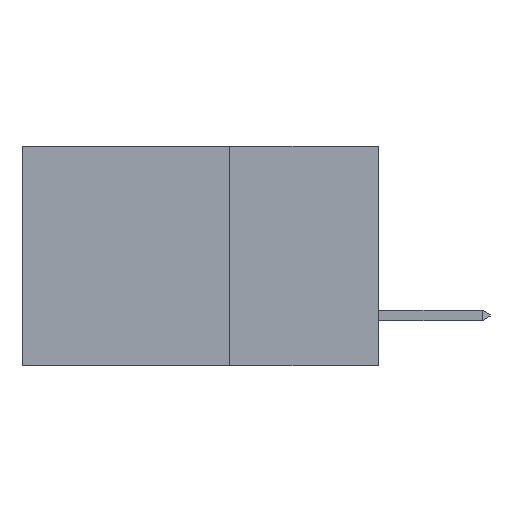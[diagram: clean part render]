
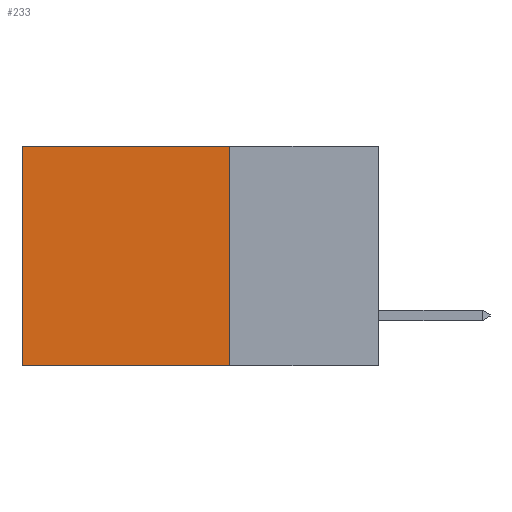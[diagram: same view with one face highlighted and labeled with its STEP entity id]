
A CAD part, left-side view. The second image highlights one B-rep face of the part: STEP entity #233.
In plain terms, the highlighted planar face has unit normal (-1, 0, 0).
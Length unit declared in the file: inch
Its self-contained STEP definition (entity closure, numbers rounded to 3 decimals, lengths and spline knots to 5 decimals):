
#233 = ADVANCED_FACE ( 'NONE', ( #6639 ), #3159, .F. ) ;
#832 = LINE ( 'NONE', #1231, #11042 ) ;
#1231 = CARTESIAN_POINT ( 'NONE',  ( 0.298, 0.25, 0. ) ) ;
#2333 = DIRECTION ( 'NONE',  ( 1., 0., 0. ) ) ;
#2542 = EDGE_LOOP ( 'NONE', ( #14086, #16759, #12512, #13040 ) ) ;
#3117 = LINE ( 'NONE', #8276, #12896 ) ;
#3159 = PLANE ( 'NONE',  #7513 ) ;
#3328 = CARTESIAN_POINT ( 'NONE',  ( 0.298, 0.25, 0. ) ) ;
#3473 = DIRECTION ( 'NONE',  ( 0., 0., -1. ) ) ;
#3909 = LINE ( 'NONE', #15933, #10576 ) ;
#3945 = DIRECTION ( 'NONE',  ( 0., 0., -1. ) ) ;
#4232 = CARTESIAN_POINT ( 'NONE',  ( 0.298, 0.6, 0. ) ) ;
#5231 = EDGE_CURVE ( 'NONE', #8974, #6561, #3909, .T. ) ;
#5378 = VECTOR ( 'NONE', #3473, 39.37008 ) ;
#5754 = EDGE_CURVE ( 'NONE', #14826, #6561, #15957, .T. ) ;
#6089 = CARTESIAN_POINT ( 'NONE',  ( 0.298, 0.25, -0.37 ) ) ;
#6561 = VERTEX_POINT ( 'NONE', #13913 ) ;
#6639 = FACE_OUTER_BOUND ( 'NONE', #2542, .T. ) ;
#7513 = AXIS2_PLACEMENT_3D ( 'NONE', #3328, #2333, #3945 ) ;
#7724 = CARTESIAN_POINT ( 'NONE',  ( 0.298, 0.25, 0. ) ) ;
#8276 = CARTESIAN_POINT ( 'NONE',  ( 0.298, 0.25, 0. ) ) ;
#8974 = VERTEX_POINT ( 'NONE', #6089 ) ;
#10576 = VECTOR ( 'NONE', #15473, 39.37008 ) ;
#11042 = VECTOR ( 'NONE', #11871, 39.37008 ) ;
#11689 = EDGE_CURVE ( 'NONE', #13024, #14826, #832, .T. ) ;
#11871 = DIRECTION ( 'NONE',  ( 0., 1., 0. ) ) ;
#12247 = DIRECTION ( 'NONE',  ( 0., 0., -1. ) ) ;
#12512 = ORIENTED_EDGE ( 'NONE', *, *, #14843, .F. ) ;
#12896 = VECTOR ( 'NONE', #12247, 39.37008 ) ;
#13024 = VERTEX_POINT ( 'NONE', #7724 ) ;
#13040 = ORIENTED_EDGE ( 'NONE', *, *, #11689, .T. ) ;
#13913 = CARTESIAN_POINT ( 'NONE',  ( 0.298, 0.6, -0.37 ) ) ;
#14086 = ORIENTED_EDGE ( 'NONE', *, *, #5754, .T. ) ;
#14826 = VERTEX_POINT ( 'NONE', #4232 ) ;
#14843 = EDGE_CURVE ( 'NONE', #13024, #8974, #3117, .T. ) ;
#15417 = CARTESIAN_POINT ( 'NONE',  ( 0.298, 0.6, 0. ) ) ;
#15473 = DIRECTION ( 'NONE',  ( 0., 1., 0. ) ) ;
#15933 = CARTESIAN_POINT ( 'NONE',  ( 0.298, 0.25, -0.37 ) ) ;
#15957 = LINE ( 'NONE', #15417, #5378 ) ;
#16759 = ORIENTED_EDGE ( 'NONE', *, *, #5231, .F. ) ;
